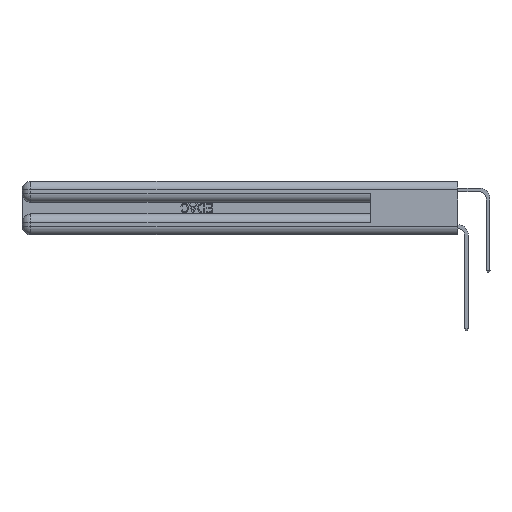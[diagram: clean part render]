
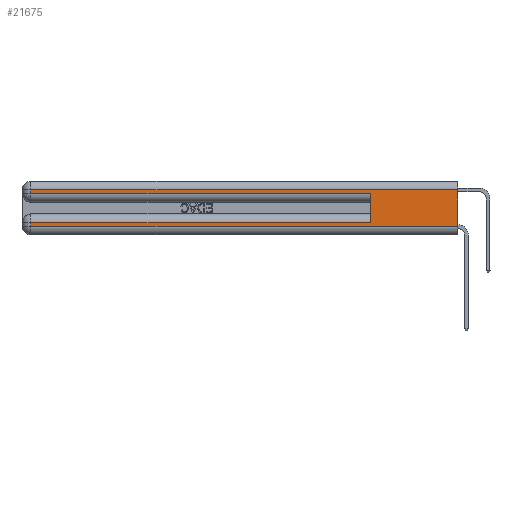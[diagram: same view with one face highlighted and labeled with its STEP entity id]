
A CAD part, left-side view. The second image highlights one B-rep face of the part: STEP entity #21675.
In plain terms, the highlighted planar face has unit normal (-1, 0, 0).
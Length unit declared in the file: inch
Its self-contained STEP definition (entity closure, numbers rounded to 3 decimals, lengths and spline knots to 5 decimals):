
#149 = CARTESIAN_POINT ( 'NONE',  ( 0., 0.6, 0.085 ) ) ;
#306 = EDGE_LOOP ( 'NONE', ( #7694, #31343, #30751, #9224, #32888, #26968, #2414, #10300 ) ) ;
#864 = CARTESIAN_POINT ( 'NONE',  ( 0., 2.94, 0.31 ) ) ;
#1856 = DIRECTION ( 'NONE',  ( 0., 0., -1. ) ) ;
#2171 = CARTESIAN_POINT ( 'NONE',  ( 0., 0., 0.285 ) ) ;
#2414 = ORIENTED_EDGE ( 'NONE', *, *, #3021, .T. ) ;
#2491 = VERTEX_POINT ( 'NONE', #18688 ) ;
#3021 = EDGE_CURVE ( 'NONE', #23084, #22419, #28729, .T. ) ;
#3294 = LINE ( 'NONE', #24186, #16861 ) ;
#3432 = LINE ( 'NONE', #27554, #30980 ) ;
#3560 = CARTESIAN_POINT ( 'NONE',  ( 0., 0., 0.06 ) ) ;
#4071 = DIRECTION ( 'NONE',  ( 1., 0., 0. ) ) ;
#5061 = EDGE_CURVE ( 'NONE', #2491, #25016, #20105, .T. ) ;
#5293 = CARTESIAN_POINT ( 'NONE',  ( 0., 2.94, 0.37 ) ) ;
#5713 = VECTOR ( 'NONE', #15727, 39.37008 ) ;
#5856 = CARTESIAN_POINT ( 'NONE',  ( 0., 2.94, 0.085 ) ) ;
#7209 = CARTESIAN_POINT ( 'NONE',  ( 0., 0., 0.06 ) ) ;
#7350 = DIRECTION ( 'NONE',  ( 0., 0., 1. ) ) ;
#7694 = ORIENTED_EDGE ( 'NONE', *, *, #9740, .F. ) ;
#8229 = EDGE_CURVE ( 'NONE', #32798, #24891, #15172, .T. ) ;
#8577 = DIRECTION ( 'NONE',  ( 0., 0., -1. ) ) ;
#8766 = CARTESIAN_POINT ( 'NONE',  ( 0., 2.94, 0.06 ) ) ;
#9149 = LINE ( 'NONE', #21996, #30608 ) ;
#9224 = ORIENTED_EDGE ( 'NONE', *, *, #8229, .T. ) ;
#9740 = EDGE_CURVE ( 'NONE', #2491, #10927, #9149, .T. ) ;
#10300 = ORIENTED_EDGE ( 'NONE', *, *, #29122, .T. ) ;
#10927 = VERTEX_POINT ( 'NONE', #3560 ) ;
#11970 = VECTOR ( 'NONE', #25354, 39.37008 ) ;
#12071 = DIRECTION ( 'NONE',  ( 0., 0., -1. ) ) ;
#12431 = DIRECTION ( 'NONE',  ( 0., -1., 0. ) ) ;
#12499 = CARTESIAN_POINT ( 'NONE',  ( 0., 0.6, 0.145 ) ) ;
#14028 = DIRECTION ( 'NONE',  ( 0., 1., 0. ) ) ;
#14844 = AXIS2_PLACEMENT_3D ( 'NONE', #33165, #4071, #1856 ) ;
#14859 = PLANE ( 'NONE',  #14844 ) ;
#15172 = LINE ( 'NONE', #2171, #26871 ) ;
#15727 = DIRECTION ( 'NONE',  ( 0., 0., -1. ) ) ;
#16861 = VECTOR ( 'NONE', #8577, 39.37008 ) ;
#18688 = CARTESIAN_POINT ( 'NONE',  ( 0., 0., 0.31 ) ) ;
#19001 = VECTOR ( 'NONE', #7350, 39.37008 ) ;
#19618 = VECTOR ( 'NONE', #24752, 39.37008 ) ;
#20032 = LINE ( 'NONE', #7209, #11970 ) ;
#20105 = LINE ( 'NONE', #22686, #19618 ) ;
#20519 = LINE ( 'NONE', #12499, #19001 ) ;
#20906 = CARTESIAN_POINT ( 'NONE',  ( 0., 0.6, 0.285 ) ) ;
#21675 = ADVANCED_FACE ( 'NONE', ( #22721 ), #14859, .F. ) ;
#21996 = CARTESIAN_POINT ( 'NONE',  ( 0., 0., 0.37 ) ) ;
#22419 = VERTEX_POINT ( 'NONE', #8766 ) ;
#22686 = CARTESIAN_POINT ( 'NONE',  ( 0., 0., 0.31 ) ) ;
#22721 = FACE_OUTER_BOUND ( 'NONE', #306, .T. ) ;
#23084 = VERTEX_POINT ( 'NONE', #5856 ) ;
#24186 = CARTESIAN_POINT ( 'NONE',  ( 0., 2.94, 0.37 ) ) ;
#24752 = DIRECTION ( 'NONE',  ( 0., 1., 0. ) ) ;
#24891 = VERTEX_POINT ( 'NONE', #20906 ) ;
#24979 = EDGE_CURVE ( 'NONE', #26725, #23084, #3432, .T. ) ;
#25016 = VERTEX_POINT ( 'NONE', #864 ) ;
#25354 = DIRECTION ( 'NONE',  ( 0., -1., 0. ) ) ;
#26725 = VERTEX_POINT ( 'NONE', #149 ) ;
#26871 = VECTOR ( 'NONE', #12431, 39.37008 ) ;
#26968 = ORIENTED_EDGE ( 'NONE', *, *, #24979, .T. ) ;
#27554 = CARTESIAN_POINT ( 'NONE',  ( 0., 0., 0.085 ) ) ;
#27874 = CARTESIAN_POINT ( 'NONE',  ( 0., 2.94, 0.285 ) ) ;
#28729 = LINE ( 'NONE', #5293, #5713 ) ;
#29051 = EDGE_CURVE ( 'NONE', #25016, #32798, #3294, .T. ) ;
#29122 = EDGE_CURVE ( 'NONE', #22419, #10927, #20032, .T. ) ;
#30608 = VECTOR ( 'NONE', #12071, 39.37008 ) ;
#30751 = ORIENTED_EDGE ( 'NONE', *, *, #29051, .T. ) ;
#30980 = VECTOR ( 'NONE', #14028, 39.37008 ) ;
#31343 = ORIENTED_EDGE ( 'NONE', *, *, #5061, .T. ) ;
#32432 = EDGE_CURVE ( 'NONE', #26725, #24891, #20519, .T. ) ;
#32798 = VERTEX_POINT ( 'NONE', #27874 ) ;
#32888 = ORIENTED_EDGE ( 'NONE', *, *, #32432, .F. ) ;
#33165 = CARTESIAN_POINT ( 'NONE',  ( 0., 0., 0.37 ) ) ;
